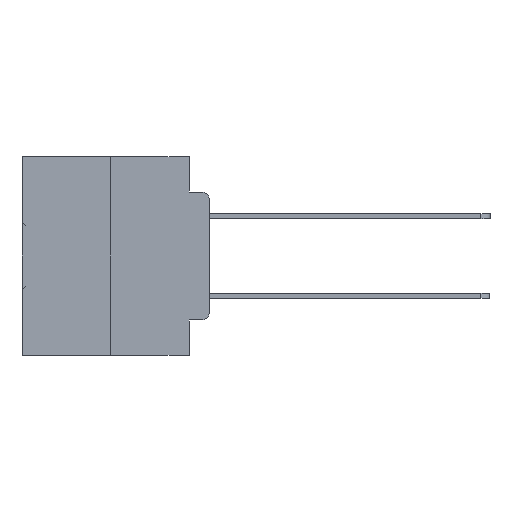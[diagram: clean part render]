
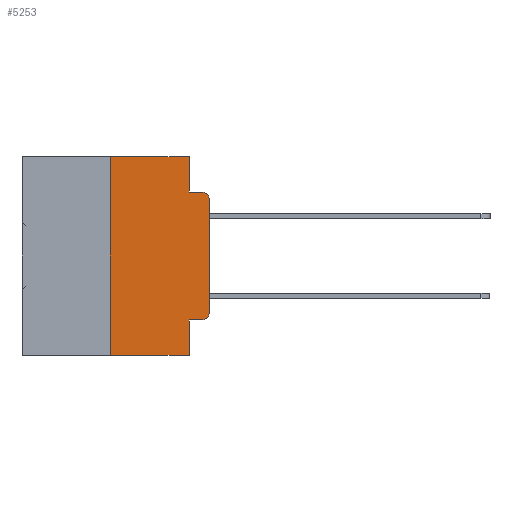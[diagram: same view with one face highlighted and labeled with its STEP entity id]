
A CAD part, left-side view. The second image highlights one B-rep face of the part: STEP entity #5253.
In plain terms, the highlighted planar face has unit normal (-1, 0, 0).
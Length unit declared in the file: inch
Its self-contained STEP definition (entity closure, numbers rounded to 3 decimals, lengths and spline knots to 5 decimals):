
#349 = EDGE_CURVE ( 'NONE', #24751, #11965, #1339, .T. ) ;
#653 = ORIENTED_EDGE ( 'NONE', *, *, #28258, .T. ) ;
#731 = CARTESIAN_POINT ( 'NONE',  ( 0., 0.051, -0.4115 ) ) ;
#946 = DIRECTION ( 'NONE',  ( -1., 0., 0. ) ) ;
#1022 = EDGE_LOOP ( 'NONE', ( #5409, #23746, #10686, #27171, #14210, #9389, #11136, #26754, #5448, #653 ) ) ;
#1064 = CIRCLE ( 'NONE', #35655, 0.02 ) ;
#1339 = LINE ( 'NONE', #29934, #8800 ) ;
#2418 = DIRECTION ( 'NONE',  ( 0., 0., 1. ) ) ;
#3350 = EDGE_CURVE ( 'NONE', #32369, #11965, #18553, .T. ) ;
#4321 = DIRECTION ( 'NONE',  ( 0., -1., 0. ) ) ;
#4518 = EDGE_CURVE ( 'NONE', #10587, #11227, #30919, .T. ) ;
#5253 = ADVANCED_FACE ( 'NONE', ( #21430 ), #33307, .F. ) ;
#5409 = ORIENTED_EDGE ( 'NONE', *, *, #4518, .T. ) ;
#5421 = VECTOR ( 'NONE', #30118, 39.37008 ) ;
#5448 = ORIENTED_EDGE ( 'NONE', *, *, #35486, .T. ) ;
#5539 = VECTOR ( 'NONE', #2418, 39.37008 ) ;
#6140 = VERTEX_POINT ( 'NONE', #34666 ) ;
#6526 = CARTESIAN_POINT ( 'NONE',  ( 0., 0.02, -0.3915 ) ) ;
#7668 = CARTESIAN_POINT ( 'NONE',  ( 0., 0.051, -0.5 ) ) ;
#8800 = VECTOR ( 'NONE', #30610, 39.37008 ) ;
#8899 = LINE ( 'NONE', #29302, #15449 ) ;
#9355 = DIRECTION ( 'NONE',  ( 0., 0., -1. ) ) ;
#9389 = ORIENTED_EDGE ( 'NONE', *, *, #18351, .F. ) ;
#9817 = CARTESIAN_POINT ( 'NONE',  ( 0., 0.25, 0. ) ) ;
#10587 = VERTEX_POINT ( 'NONE', #28961 ) ;
#10686 = ORIENTED_EDGE ( 'NONE', *, *, #27569, .F. ) ;
#10793 = CARTESIAN_POINT ( 'NONE',  ( 0., 0.051, 0. ) ) ;
#10857 = AXIS2_PLACEMENT_3D ( 'NONE', #6526, #25996, #9355 ) ;
#11136 = ORIENTED_EDGE ( 'NONE', *, *, #349, .T. ) ;
#11227 = VERTEX_POINT ( 'NONE', #32123 ) ;
#11402 = DIRECTION ( 'NONE',  ( 1., 0., 0. ) ) ;
#11965 = VERTEX_POINT ( 'NONE', #7668 ) ;
#12008 = CARTESIAN_POINT ( 'NONE',  ( 0., 0.051, 0. ) ) ;
#12532 = VECTOR ( 'NONE', #22660, 39.37008 ) ;
#13564 = DIRECTION ( 'NONE',  ( 0., 0., -1. ) ) ;
#13791 = DIRECTION ( 'NONE',  ( 0., 0., 1. ) ) ;
#14210 = ORIENTED_EDGE ( 'NONE', *, *, #32655, .F. ) ;
#14426 = CARTESIAN_POINT ( 'NONE',  ( 0., 0.051, -0.0885 ) ) ;
#14531 = VECTOR ( 'NONE', #13564, 39.37008 ) ;
#15449 = VECTOR ( 'NONE', #4321, 39.37008 ) ;
#16463 = LINE ( 'NONE', #29938, #23843 ) ;
#17702 = CARTESIAN_POINT ( 'NONE',  ( 0., 0.02, -0.1085 ) ) ;
#18351 = EDGE_CURVE ( 'NONE', #24751, #31378, #20408, .T. ) ;
#18553 = LINE ( 'NONE', #10793, #5421 ) ;
#19442 = CIRCLE ( 'NONE', #10857, 0.02 ) ;
#19703 = CARTESIAN_POINT ( 'NONE',  ( 0., 0.473, 0. ) ) ;
#20177 = AXIS2_PLACEMENT_3D ( 'NONE', #19703, #11402, #30722 ) ;
#20408 = LINE ( 'NONE', #35516, #5539 ) ;
#20503 = DIRECTION ( 'NONE',  ( 0., 0., -1. ) ) ;
#21430 = FACE_OUTER_BOUND ( 'NONE', #1022, .T. ) ;
#21694 = DIRECTION ( 'NONE',  ( 0., -1., 0. ) ) ;
#22199 = VERTEX_POINT ( 'NONE', #30530 ) ;
#22494 = VERTEX_POINT ( 'NONE', #23595 ) ;
#22660 = DIRECTION ( 'NONE',  ( 0., -1., 0. ) ) ;
#23595 = CARTESIAN_POINT ( 'NONE',  ( 0., 0.02, -0.0885 ) ) ;
#23746 = ORIENTED_EDGE ( 'NONE', *, *, #34814, .T. ) ;
#23843 = VECTOR ( 'NONE', #21694, 39.37008 ) ;
#23908 = EDGE_CURVE ( 'NONE', #26906, #6140, #35509, .T. ) ;
#24751 = VERTEX_POINT ( 'NONE', #35767 ) ;
#25996 = DIRECTION ( 'NONE',  ( -1., 0., 0. ) ) ;
#26754 = ORIENTED_EDGE ( 'NONE', *, *, #3350, .F. ) ;
#26906 = VERTEX_POINT ( 'NONE', #12008 ) ;
#27171 = ORIENTED_EDGE ( 'NONE', *, *, #23908, .F. ) ;
#27227 = LINE ( 'NONE', #14426, #12532 ) ;
#27569 = EDGE_CURVE ( 'NONE', #6140, #22494, #27227, .T. ) ;
#28258 = EDGE_CURVE ( 'NONE', #22199, #10587, #19442, .T. ) ;
#28961 = CARTESIAN_POINT ( 'NONE',  ( 0., 0., -0.3915 ) ) ;
#29302 = CARTESIAN_POINT ( 'NONE',  ( 0., 0.051, -0.4115 ) ) ;
#29934 = CARTESIAN_POINT ( 'NONE',  ( 0., 0.473, -0.5 ) ) ;
#29938 = CARTESIAN_POINT ( 'NONE',  ( 0., 0.473, 0. ) ) ;
#30057 = CARTESIAN_POINT ( 'NONE',  ( 0., 0.051, 0. ) ) ;
#30118 = DIRECTION ( 'NONE',  ( 0., 0., -1. ) ) ;
#30291 = CARTESIAN_POINT ( 'NONE',  ( 0., 0., 0. ) ) ;
#30530 = CARTESIAN_POINT ( 'NONE',  ( 0., 0.02, -0.4115 ) ) ;
#30610 = DIRECTION ( 'NONE',  ( 0., -1., 0. ) ) ;
#30722 = DIRECTION ( 'NONE',  ( 0., 0., -1. ) ) ;
#30919 = LINE ( 'NONE', #30291, #32600 ) ;
#31378 = VERTEX_POINT ( 'NONE', #9817 ) ;
#32123 = CARTESIAN_POINT ( 'NONE',  ( 0., 0., -0.1085 ) ) ;
#32369 = VERTEX_POINT ( 'NONE', #731 ) ;
#32600 = VECTOR ( 'NONE', #13791, 39.37008 ) ;
#32655 = EDGE_CURVE ( 'NONE', #31378, #26906, #16463, .T. ) ;
#33307 = PLANE ( 'NONE',  #20177 ) ;
#34666 = CARTESIAN_POINT ( 'NONE',  ( 0., 0.051, -0.0885 ) ) ;
#34814 = EDGE_CURVE ( 'NONE', #11227, #22494, #1064, .T. ) ;
#35486 = EDGE_CURVE ( 'NONE', #32369, #22199, #8899, .T. ) ;
#35509 = LINE ( 'NONE', #30057, #14531 ) ;
#35516 = CARTESIAN_POINT ( 'NONE',  ( 0., 0.25, 0. ) ) ;
#35655 = AXIS2_PLACEMENT_3D ( 'NONE', #17702, #946, #20503 ) ;
#35767 = CARTESIAN_POINT ( 'NONE',  ( 0., 0.25, -0.5 ) ) ;
